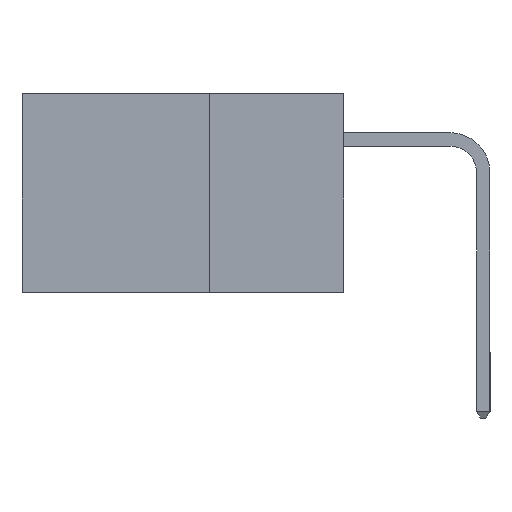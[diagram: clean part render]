
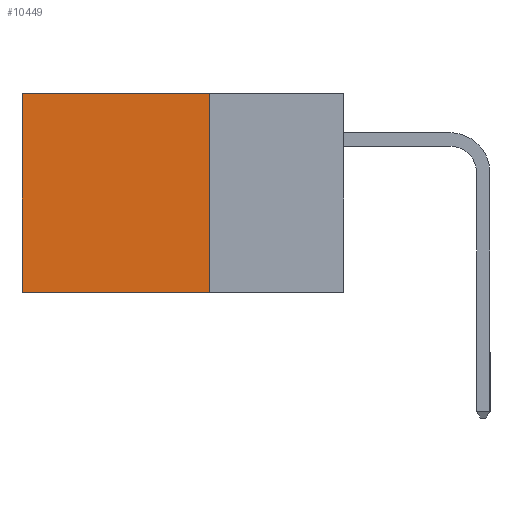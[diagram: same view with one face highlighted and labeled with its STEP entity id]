
A CAD part, left-side view. The second image highlights one B-rep face of the part: STEP entity #10449.
In plain terms, the highlighted planar face has unit normal (-1, 0, 0).
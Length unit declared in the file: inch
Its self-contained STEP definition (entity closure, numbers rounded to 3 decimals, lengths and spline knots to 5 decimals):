
#145 = ORIENTED_EDGE ( 'NONE', *, *, #17003, .F. ) ;
#1296 = DIRECTION ( 'NONE',  ( 1., 0., 0. ) ) ;
#1502 = VERTEX_POINT ( 'NONE', #6422 ) ;
#1752 = EDGE_CURVE ( 'NONE', #1502, #3783, #9780, .T. ) ;
#3163 = CARTESIAN_POINT ( 'NONE',  ( 0.2615, 0.6, -0.37 ) ) ;
#3783 = VERTEX_POINT ( 'NONE', #3163 ) ;
#3909 = DIRECTION ( 'NONE',  ( 0., 0., -1. ) ) ;
#3989 = FACE_OUTER_BOUND ( 'NONE', #15142, .T. ) ;
#4415 = CARTESIAN_POINT ( 'NONE',  ( 0.2615, 0.6, -0.37 ) ) ;
#4982 = VECTOR ( 'NONE', #5531, 39.37008 ) ;
#5162 = VECTOR ( 'NONE', #15431, 39.37008 ) ;
#5284 = CARTESIAN_POINT ( 'NONE',  ( 0.2615, 0.25, -0.37 ) ) ;
#5531 = DIRECTION ( 'NONE',  ( 0., 1., 0. ) ) ;
#5611 = CARTESIAN_POINT ( 'NONE',  ( 0.2615, 0.25, -0.37 ) ) ;
#5854 = VERTEX_POINT ( 'NONE', #8339 ) ;
#6060 = CARTESIAN_POINT ( 'NONE',  ( 0.2615, 0.25, -0.37 ) ) ;
#6422 = CARTESIAN_POINT ( 'NONE',  ( 0.2615, 0.6, 0. ) ) ;
#6521 = CARTESIAN_POINT ( 'NONE',  ( 0.2615, 0.25, 0. ) ) ;
#8245 = VERTEX_POINT ( 'NONE', #12062 ) ;
#8339 = CARTESIAN_POINT ( 'NONE',  ( 0.2615, 0.25, 0. ) ) ;
#8481 = DIRECTION ( 'NONE',  ( 0., 0., -1. ) ) ;
#9275 = EDGE_CURVE ( 'NONE', #8245, #3783, #13644, .T. ) ;
#9780 = LINE ( 'NONE', #4415, #14824 ) ;
#10143 = ORIENTED_EDGE ( 'NONE', *, *, #1752, .T. ) ;
#10449 = ADVANCED_FACE ( 'NONE', ( #3989 ), #12988, .F. ) ;
#10716 = VECTOR ( 'NONE', #16856, 39.37008 ) ;
#11514 = LINE ( 'NONE', #6060, #10716 ) ;
#11637 = LINE ( 'NONE', #6521, #5162 ) ;
#12062 = CARTESIAN_POINT ( 'NONE',  ( 0.2615, 0.25, -0.37 ) ) ;
#12116 = ORIENTED_EDGE ( 'NONE', *, *, #16411, .T. ) ;
#12988 = PLANE ( 'NONE',  #15518 ) ;
#13644 = LINE ( 'NONE', #5611, #4982 ) ;
#14824 = VECTOR ( 'NONE', #8481, 39.37008 ) ;
#15142 = EDGE_LOOP ( 'NONE', ( #10143, #15450, #145, #12116 ) ) ;
#15431 = DIRECTION ( 'NONE',  ( 0., 1., 0. ) ) ;
#15450 = ORIENTED_EDGE ( 'NONE', *, *, #9275, .F. ) ;
#15518 = AXIS2_PLACEMENT_3D ( 'NONE', #5284, #1296, #3909 ) ;
#16411 = EDGE_CURVE ( 'NONE', #5854, #1502, #11637, .T. ) ;
#16856 = DIRECTION ( 'NONE',  ( 0., 0., -1. ) ) ;
#17003 = EDGE_CURVE ( 'NONE', #5854, #8245, #11514, .T. ) ;
